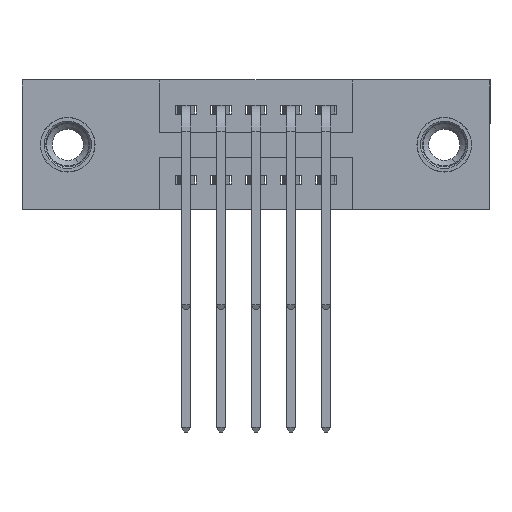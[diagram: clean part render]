
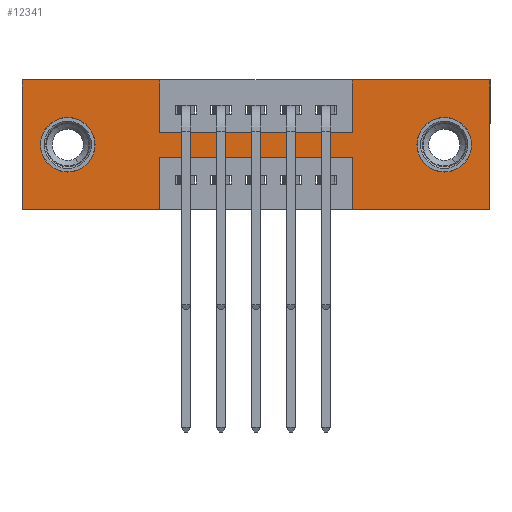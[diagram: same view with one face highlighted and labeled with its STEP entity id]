
A CAD part, front view. The second image highlights one B-rep face of the part: STEP entity #12341.
In plain terms, the highlighted planar face has unit normal (0, -1, 0).
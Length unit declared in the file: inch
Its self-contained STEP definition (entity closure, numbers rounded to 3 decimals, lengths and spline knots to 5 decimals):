
#30 = CARTESIAN_POINT ( 'NONE',  ( 0.3925, 0., -0.15 ) ) ;
#41 = ORIENTED_EDGE ( 'NONE', *, *, #13207, .F. ) ;
#99 = EDGE_CURVE ( 'NONE', #1684, #14518, #3816, .T. ) ;
#213 = DIRECTION ( 'NONE',  ( -1., 0., 0. ) ) ;
#618 = VERTEX_POINT ( 'NONE', #7897 ) ;
#759 = EDGE_LOOP ( 'NONE', ( #9100, #14108 ) ) ;
#891 = DIRECTION ( 'NONE',  ( 0., -1., 0. ) ) ;
#950 = CIRCLE ( 'NONE', #6288, 0.078 ) ;
#1003 = EDGE_CURVE ( 'NONE', #618, #1684, #4948, .T. ) ;
#1112 = CARTESIAN_POINT ( 'NONE',  ( 0., 0., -0.37 ) ) ;
#1121 = EDGE_CURVE ( 'NONE', #5391, #14096, #3783, .T. ) ;
#1199 = EDGE_CURVE ( 'NONE', #14518, #6940, #2640, .T. ) ;
#1380 = VECTOR ( 'NONE', #9141, 39.37008 ) ;
#1387 = CARTESIAN_POINT ( 'NONE',  ( 0.3925, 0., -0.22 ) ) ;
#1455 = LINE ( 'NONE', #14220, #13977 ) ;
#1476 = ORIENTED_EDGE ( 'NONE', *, *, #12130, .F. ) ;
#1618 = CARTESIAN_POINT ( 'NONE',  ( 0., 0., 0. ) ) ;
#1684 = VERTEX_POINT ( 'NONE', #6230 ) ;
#1841 = EDGE_CURVE ( 'NONE', #12496, #14737, #8449, .T. ) ;
#1917 = CARTESIAN_POINT ( 'NONE',  ( 0., 0., 0. ) ) ;
#1934 = CIRCLE ( 'NONE', #3381, 0.078 ) ;
#2310 = DIRECTION ( 'NONE',  ( 0., 1., 0. ) ) ;
#2640 = LINE ( 'NONE', #4575, #9174 ) ;
#2668 = VECTOR ( 'NONE', #12979, 39.37008 ) ;
#2695 = ORIENTED_EDGE ( 'NONE', *, *, #11501, .F. ) ;
#2762 = ORIENTED_EDGE ( 'NONE', *, *, #1003, .F. ) ;
#2850 = AXIS2_PLACEMENT_3D ( 'NONE', #3343, #10267, #3483 ) ;
#3102 = CARTESIAN_POINT ( 'NONE',  ( 0.3925, 0., 0. ) ) ;
#3108 = VERTEX_POINT ( 'NONE', #10490 ) ;
#3266 = FACE_OUTER_BOUND ( 'NONE', #7260, .T. ) ;
#3343 = CARTESIAN_POINT ( 'NONE',  ( 1.205, 0., -0.185 ) ) ;
#3381 = AXIS2_PLACEMENT_3D ( 'NONE', #3564, #11638, #4801 ) ;
#3483 = DIRECTION ( 'NONE',  ( 0., 0., -1. ) ) ;
#3547 = CARTESIAN_POINT ( 'NONE',  ( 0.9425, 0., -0.37 ) ) ;
#3564 = CARTESIAN_POINT ( 'NONE',  ( 1.205, 0., -0.185 ) ) ;
#3652 = CARTESIAN_POINT ( 'NONE',  ( 0.3925, 0., -0.37 ) ) ;
#3783 = LINE ( 'NONE', #1387, #4185 ) ;
#3816 = LINE ( 'NONE', #6696, #2668 ) ;
#3817 = VECTOR ( 'NONE', #10370, 39.37008 ) ;
#3865 = ORIENTED_EDGE ( 'NONE', *, *, #1121, .F. ) ;
#4185 = VECTOR ( 'NONE', #213, 39.37008 ) ;
#4575 = CARTESIAN_POINT ( 'NONE',  ( 0., 0., -0.37 ) ) ;
#4681 = VECTOR ( 'NONE', #13179, 39.37008 ) ;
#4742 = EDGE_CURVE ( 'NONE', #14737, #12496, #1934, .T. ) ;
#4788 = LINE ( 'NONE', #11055, #13261 ) ;
#4801 = DIRECTION ( 'NONE',  ( 0., 0., -1. ) ) ;
#4882 = DIRECTION ( 'NONE',  ( -1., 0., 0. ) ) ;
#4948 = LINE ( 'NONE', #12034, #7934 ) ;
#5129 = CARTESIAN_POINT ( 'NONE',  ( 0., 0., 0. ) ) ;
#5186 = DIRECTION ( 'NONE',  ( 0., 0., 1. ) ) ;
#5273 = CARTESIAN_POINT ( 'NONE',  ( 1.335, 0., -0.37 ) ) ;
#5378 = DIRECTION ( 'NONE',  ( -1., 0., 0. ) ) ;
#5391 = VERTEX_POINT ( 'NONE', #7138 ) ;
#5404 = VERTEX_POINT ( 'NONE', #3652 ) ;
#5622 = CARTESIAN_POINT ( 'NONE',  ( 0.13, 0., -0.185 ) ) ;
#5815 = PLANE ( 'NONE',  #6523 ) ;
#6105 = CARTESIAN_POINT ( 'NONE',  ( 1.205, 0., -0.263 ) ) ;
#6230 = CARTESIAN_POINT ( 'NONE',  ( 1.335, 0., 0. ) ) ;
#6288 = AXIS2_PLACEMENT_3D ( 'NONE', #9289, #2310, #10468 ) ;
#6476 = VERTEX_POINT ( 'NONE', #8215 ) ;
#6523 = AXIS2_PLACEMENT_3D ( 'NONE', #6923, #891, #9215 ) ;
#6696 = CARTESIAN_POINT ( 'NONE',  ( 1.335, 0., 0. ) ) ;
#6742 = DIRECTION ( 'NONE',  ( 0., 0., 1. ) ) ;
#6841 = ORIENTED_EDGE ( 'NONE', *, *, #15000, .T. ) ;
#6842 = EDGE_CURVE ( 'NONE', #14096, #5404, #7359, .T. ) ;
#6858 = CARTESIAN_POINT ( 'NONE',  ( 0.3925, 0., -0.37 ) ) ;
#6895 = LINE ( 'NONE', #13864, #3817 ) ;
#6919 = EDGE_CURVE ( 'NONE', #9330, #10544, #950, .T. ) ;
#6923 = CARTESIAN_POINT ( 'NONE',  ( 0., 0., -0.37 ) ) ;
#6940 = VERTEX_POINT ( 'NONE', #3547 ) ;
#7086 = ORIENTED_EDGE ( 'NONE', *, *, #6919, .T. ) ;
#7138 = CARTESIAN_POINT ( 'NONE',  ( 0.9425, 0., -0.22 ) ) ;
#7253 = DIRECTION ( 'NONE',  ( 0., 0., 1. ) ) ;
#7260 = EDGE_LOOP ( 'NONE', ( #12129, #3865, #41, #14164, #9269, #2762, #2695, #11118, #1476, #13868, #9522, #12154 ) ) ;
#7359 = LINE ( 'NONE', #6858, #1380 ) ;
#7693 = LINE ( 'NONE', #5129, #4681 ) ;
#7770 = CARTESIAN_POINT ( 'NONE',  ( 0.13, 0., -0.263 ) ) ;
#7776 = EDGE_CURVE ( 'NONE', #13882, #6476, #7693, .T. ) ;
#7897 = CARTESIAN_POINT ( 'NONE',  ( 0.9425, 0., 0. ) ) ;
#7934 = VECTOR ( 'NONE', #8188, 39.37008 ) ;
#7952 = LINE ( 'NONE', #1917, #14515 ) ;
#8188 = DIRECTION ( 'NONE',  ( 1., 0., 0. ) ) ;
#8215 = CARTESIAN_POINT ( 'NONE',  ( 0.3925, 0., 0. ) ) ;
#8449 = CIRCLE ( 'NONE', #2850, 0.078 ) ;
#8865 = DIRECTION ( 'NONE',  ( 0., 0., -1. ) ) ;
#8896 = VERTEX_POINT ( 'NONE', #30 ) ;
#9100 = ORIENTED_EDGE ( 'NONE', *, *, #4742, .T. ) ;
#9141 = DIRECTION ( 'NONE',  ( 0., 0., -1. ) ) ;
#9166 = VERTEX_POINT ( 'NONE', #1112 ) ;
#9174 = VECTOR ( 'NONE', #4882, 39.37008 ) ;
#9215 = DIRECTION ( 'NONE',  ( 0., 0., -1. ) ) ;
#9269 = ORIENTED_EDGE ( 'NONE', *, *, #99, .F. ) ;
#9289 = CARTESIAN_POINT ( 'NONE',  ( 0.13, 0., -0.185 ) ) ;
#9330 = VERTEX_POINT ( 'NONE', #13400 ) ;
#9522 = ORIENTED_EDGE ( 'NONE', *, *, #13436, .F. ) ;
#9697 = CARTESIAN_POINT ( 'NONE',  ( 0.9425, 0., 0. ) ) ;
#9794 = FACE_BOUND ( 'NONE', #759, .T. ) ;
#10115 = DIRECTION ( 'NONE',  ( 0., 0., 1. ) ) ;
#10267 = DIRECTION ( 'NONE',  ( 0., 1., 0. ) ) ;
#10348 = VECTOR ( 'NONE', #5186, 39.37008 ) ;
#10370 = DIRECTION ( 'NONE',  ( 1., 0., 0. ) ) ;
#10438 = EDGE_CURVE ( 'NONE', #5404, #9166, #4788, .T. ) ;
#10468 = DIRECTION ( 'NONE',  ( 0., 0., 1. ) ) ;
#10490 = CARTESIAN_POINT ( 'NONE',  ( 0.9425, 0., -0.15 ) ) ;
#10544 = VERTEX_POINT ( 'NONE', #7770 ) ;
#11055 = CARTESIAN_POINT ( 'NONE',  ( 0., 0., -0.37 ) ) ;
#11118 = ORIENTED_EDGE ( 'NONE', *, *, #13023, .F. ) ;
#11230 = VECTOR ( 'NONE', #8865, 39.37008 ) ;
#11244 = AXIS2_PLACEMENT_3D ( 'NONE', #5622, #13686, #6742 ) ;
#11501 = EDGE_CURVE ( 'NONE', #3108, #618, #13493, .T. ) ;
#11638 = DIRECTION ( 'NONE',  ( 0., 1., 0. ) ) ;
#12034 = CARTESIAN_POINT ( 'NONE',  ( 0., 0., 0. ) ) ;
#12129 = ORIENTED_EDGE ( 'NONE', *, *, #6842, .F. ) ;
#12130 = EDGE_CURVE ( 'NONE', #6476, #8896, #14710, .T. ) ;
#12154 = ORIENTED_EDGE ( 'NONE', *, *, #10438, .F. ) ;
#12155 = FACE_BOUND ( 'NONE', #14344, .T. ) ;
#12341 = ADVANCED_FACE ( 'NONE', ( #9794, #12155, #3266 ), #5815, .T. ) ;
#12496 = VERTEX_POINT ( 'NONE', #6105 ) ;
#12979 = DIRECTION ( 'NONE',  ( 0., 0., -1. ) ) ;
#13023 = EDGE_CURVE ( 'NONE', #8896, #3108, #6895, .T. ) ;
#13084 = CARTESIAN_POINT ( 'NONE',  ( 1.205, 0., -0.107 ) ) ;
#13179 = DIRECTION ( 'NONE',  ( 1., 0., 0. ) ) ;
#13207 = EDGE_CURVE ( 'NONE', #6940, #5391, #1455, .T. ) ;
#13222 = CIRCLE ( 'NONE', #11244, 0.078 ) ;
#13261 = VECTOR ( 'NONE', #5378, 39.37008 ) ;
#13400 = CARTESIAN_POINT ( 'NONE',  ( 0.13, 0., -0.107 ) ) ;
#13436 = EDGE_CURVE ( 'NONE', #9166, #13882, #7952, .T. ) ;
#13493 = LINE ( 'NONE', #9697, #10348 ) ;
#13686 = DIRECTION ( 'NONE',  ( 0., 1., 0. ) ) ;
#13746 = CARTESIAN_POINT ( 'NONE',  ( 0.3925, 0., -0.22 ) ) ;
#13864 = CARTESIAN_POINT ( 'NONE',  ( 0.3925, 0., -0.15 ) ) ;
#13868 = ORIENTED_EDGE ( 'NONE', *, *, #7776, .F. ) ;
#13882 = VERTEX_POINT ( 'NONE', #1618 ) ;
#13977 = VECTOR ( 'NONE', #7253, 39.37008 ) ;
#14096 = VERTEX_POINT ( 'NONE', #13746 ) ;
#14108 = ORIENTED_EDGE ( 'NONE', *, *, #1841, .T. ) ;
#14164 = ORIENTED_EDGE ( 'NONE', *, *, #1199, .F. ) ;
#14220 = CARTESIAN_POINT ( 'NONE',  ( 0.9425, 0., -0.37 ) ) ;
#14344 = EDGE_LOOP ( 'NONE', ( #7086, #6841 ) ) ;
#14515 = VECTOR ( 'NONE', #10115, 39.37008 ) ;
#14518 = VERTEX_POINT ( 'NONE', #5273 ) ;
#14710 = LINE ( 'NONE', #3102, #11230 ) ;
#14737 = VERTEX_POINT ( 'NONE', #13084 ) ;
#15000 = EDGE_CURVE ( 'NONE', #10544, #9330, #13222, .T. ) ;
